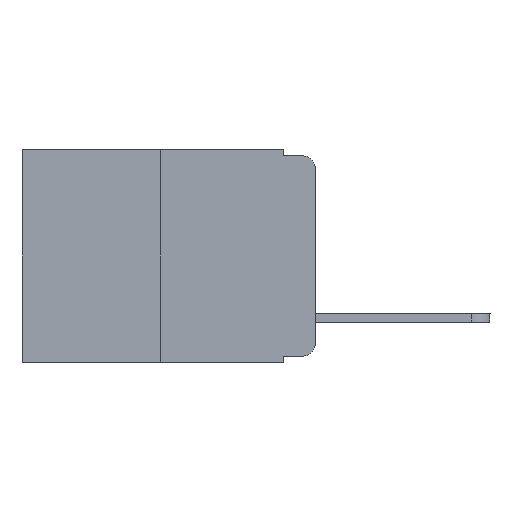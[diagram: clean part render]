
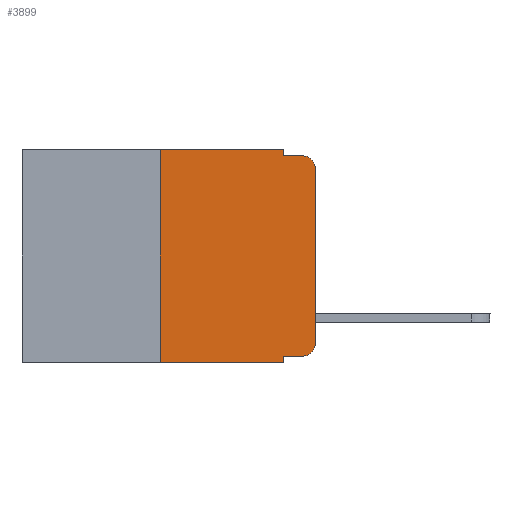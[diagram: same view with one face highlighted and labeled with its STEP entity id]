
A CAD part, left-side view. The second image highlights one B-rep face of the part: STEP entity #3899.
In plain terms, the highlighted planar face has unit normal (-1, 0, 0).
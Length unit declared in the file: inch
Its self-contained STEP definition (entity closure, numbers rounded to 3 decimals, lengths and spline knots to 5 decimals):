
#69 = DIRECTION ( 'NONE',  ( 0., 0., -1. ) ) ;
#174 = VECTOR ( 'NONE', #3391, 39.37008 ) ;
#412 = LINE ( 'NONE', #1487, #5957 ) ;
#480 = CARTESIAN_POINT ( 'NONE',  ( 0., 0.051, 0. ) ) ;
#565 = CARTESIAN_POINT ( 'NONE',  ( 0., 0., -0.03 ) ) ;
#623 = AXIS2_PLACEMENT_3D ( 'NONE', #11906, #13900, #8279 ) ;
#658 = LINE ( 'NONE', #15316, #20603 ) ;
#960 = ORIENTED_EDGE ( 'NONE', *, *, #9720, .F. ) ;
#1487 = CARTESIAN_POINT ( 'NONE',  ( 0., 0., 0. ) ) ;
#1851 = DIRECTION ( 'NONE',  ( 0., -1., 0. ) ) ;
#2114 = CARTESIAN_POINT ( 'NONE',  ( 0., 0.02, -0.03 ) ) ;
#2610 = CARTESIAN_POINT ( 'NONE',  ( 0., 0.051, 0. ) ) ;
#2783 = DIRECTION ( 'NONE',  ( 0., 0., -1. ) ) ;
#3284 = DIRECTION ( 'NONE',  ( 0., 0., 1. ) ) ;
#3391 = DIRECTION ( 'NONE',  ( 0., -1., 0. ) ) ;
#3551 = VERTEX_POINT ( 'NONE', #16045 ) ;
#3806 = CARTESIAN_POINT ( 'NONE',  ( 0., 0.473, -0.343 ) ) ;
#3899 = ADVANCED_FACE ( 'NONE', ( #17344 ), #12067, .F. ) ;
#4895 = CARTESIAN_POINT ( 'NONE',  ( 0., 0.02, -0.01 ) ) ;
#5018 = LINE ( 'NONE', #3806, #8516 ) ;
#5177 = CARTESIAN_POINT ( 'NONE',  ( 0., 0., -0.313 ) ) ;
#5470 = VERTEX_POINT ( 'NONE', #480 ) ;
#5683 = EDGE_CURVE ( 'NONE', #5470, #7411, #7127, .T. ) ;
#5957 = VECTOR ( 'NONE', #3284, 39.37008 ) ;
#6040 = DIRECTION ( 'NONE',  ( 0., 0., -1. ) ) ;
#7064 = VERTEX_POINT ( 'NONE', #16412 ) ;
#7068 = LINE ( 'NONE', #7978, #12544 ) ;
#7116 = CARTESIAN_POINT ( 'NONE',  ( 0., 0.051, -0.01 ) ) ;
#7127 = LINE ( 'NONE', #2610, #9449 ) ;
#7411 = VERTEX_POINT ( 'NONE', #12036 ) ;
#7890 = ORIENTED_EDGE ( 'NONE', *, *, #22062, .F. ) ;
#7978 = CARTESIAN_POINT ( 'NONE',  ( 0., 0.051, -0.333 ) ) ;
#8237 = EDGE_CURVE ( 'NONE', #23149, #22782, #10213, .T. ) ;
#8279 = DIRECTION ( 'NONE',  ( 0., 0., -1. ) ) ;
#8516 = VECTOR ( 'NONE', #1851, 39.37008 ) ;
#8551 = CARTESIAN_POINT ( 'NONE',  ( 0., 0.051, -0.343 ) ) ;
#9449 = VECTOR ( 'NONE', #2783, 39.37008 ) ;
#9564 = ORIENTED_EDGE ( 'NONE', *, *, #8237, .T. ) ;
#9720 = EDGE_CURVE ( 'NONE', #7064, #5470, #19882, .T. ) ;
#9788 = DIRECTION ( 'NONE',  ( 0., -1., 0. ) ) ;
#9961 = CARTESIAN_POINT ( 'NONE',  ( 0., 0.473, 0. ) ) ;
#10143 = VERTEX_POINT ( 'NONE', #12497 ) ;
#10213 = CIRCLE ( 'NONE', #19535, 0.02 ) ;
#10396 = ORIENTED_EDGE ( 'NONE', *, *, #11106, .T. ) ;
#10424 = AXIS2_PLACEMENT_3D ( 'NONE', #17015, #20848, #6040 ) ;
#11106 = EDGE_CURVE ( 'NONE', #16018, #23149, #412, .T. ) ;
#11569 = EDGE_CURVE ( 'NONE', #10143, #21827, #5018, .T. ) ;
#11906 = CARTESIAN_POINT ( 'NONE',  ( 0., 0.473, 0. ) ) ;
#12036 = CARTESIAN_POINT ( 'NONE',  ( 0., 0.051, -0.01 ) ) ;
#12067 = PLANE ( 'NONE',  #623 ) ;
#12497 = CARTESIAN_POINT ( 'NONE',  ( 0., 0.25, -0.343 ) ) ;
#12544 = VECTOR ( 'NONE', #15269, 39.37008 ) ;
#13175 = DIRECTION ( 'NONE',  ( -1., 0., 0. ) ) ;
#13418 = VERTEX_POINT ( 'NONE', #23629 ) ;
#13870 = ORIENTED_EDGE ( 'NONE', *, *, #23240, .T. ) ;
#13900 = DIRECTION ( 'NONE',  ( 1., 0., 0. ) ) ;
#14458 = EDGE_LOOP ( 'NONE', ( #10396, #9564, #22642, #17822, #960, #14674, #22010, #7890, #16244, #13870 ) ) ;
#14674 = ORIENTED_EDGE ( 'NONE', *, *, #22890, .F. ) ;
#14904 = LINE ( 'NONE', #7116, #174 ) ;
#14960 = VECTOR ( 'NONE', #9788, 39.37008 ) ;
#15118 = EDGE_CURVE ( 'NONE', #7411, #22782, #14904, .T. ) ;
#15269 = DIRECTION ( 'NONE',  ( 0., -1., 0. ) ) ;
#15316 = CARTESIAN_POINT ( 'NONE',  ( 0., 0.051, 0. ) ) ;
#16018 = VERTEX_POINT ( 'NONE', #5177 ) ;
#16045 = CARTESIAN_POINT ( 'NONE',  ( 0., 0.051, -0.333 ) ) ;
#16244 = ORIENTED_EDGE ( 'NONE', *, *, #23144, .T. ) ;
#16412 = CARTESIAN_POINT ( 'NONE',  ( 0., 0.25, 0. ) ) ;
#17015 = CARTESIAN_POINT ( 'NONE',  ( 0., 0.02, -0.313 ) ) ;
#17344 = FACE_OUTER_BOUND ( 'NONE', #14458, .T. ) ;
#17822 = ORIENTED_EDGE ( 'NONE', *, *, #5683, .F. ) ;
#18290 = CIRCLE ( 'NONE', #10424, 0.02 ) ;
#18331 = DIRECTION ( 'NONE',  ( 0., 0., 1. ) ) ;
#19535 = AXIS2_PLACEMENT_3D ( 'NONE', #2114, #13175, #69 ) ;
#19882 = LINE ( 'NONE', #9961, #14960 ) ;
#20603 = VECTOR ( 'NONE', #22854, 39.37008 ) ;
#20848 = DIRECTION ( 'NONE',  ( -1., 0., 0. ) ) ;
#21517 = VECTOR ( 'NONE', #18331, 39.37008 ) ;
#21827 = VERTEX_POINT ( 'NONE', #8551 ) ;
#22010 = ORIENTED_EDGE ( 'NONE', *, *, #11569, .T. ) ;
#22062 = EDGE_CURVE ( 'NONE', #3551, #21827, #658, .T. ) ;
#22642 = ORIENTED_EDGE ( 'NONE', *, *, #15118, .F. ) ;
#22782 = VERTEX_POINT ( 'NONE', #4895 ) ;
#22854 = DIRECTION ( 'NONE',  ( 0., 0., -1. ) ) ;
#22890 = EDGE_CURVE ( 'NONE', #10143, #7064, #22968, .T. ) ;
#22968 = LINE ( 'NONE', #23371, #21517 ) ;
#23144 = EDGE_CURVE ( 'NONE', #3551, #13418, #7068, .T. ) ;
#23149 = VERTEX_POINT ( 'NONE', #565 ) ;
#23240 = EDGE_CURVE ( 'NONE', #13418, #16018, #18290, .T. ) ;
#23371 = CARTESIAN_POINT ( 'NONE',  ( 0., 0.25, 0. ) ) ;
#23629 = CARTESIAN_POINT ( 'NONE',  ( 0., 0.02, -0.333 ) ) ;
